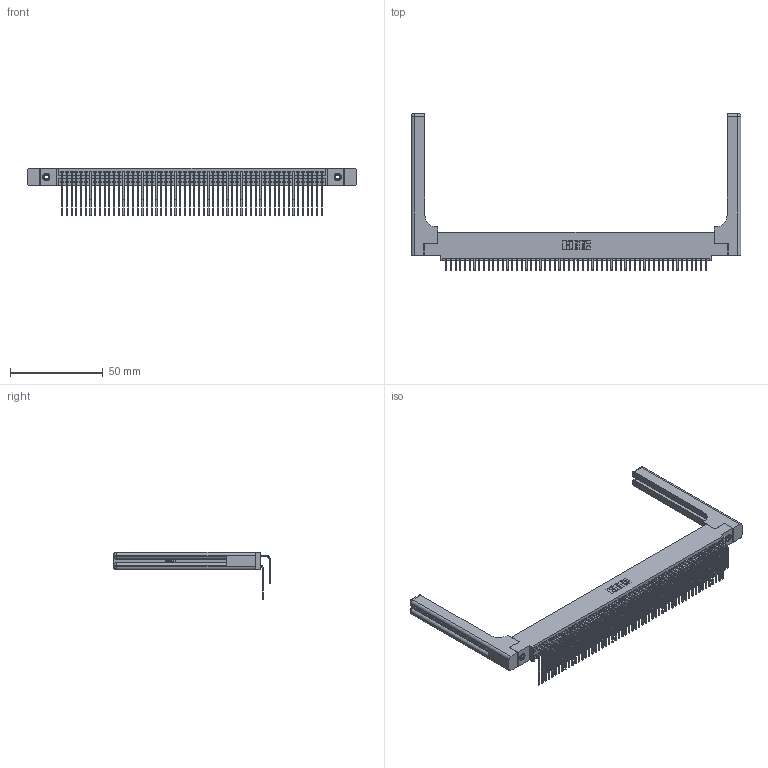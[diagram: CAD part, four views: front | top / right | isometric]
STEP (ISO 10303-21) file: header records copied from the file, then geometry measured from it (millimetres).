
FILE_DESCRIPTION (( 'STEP AP203' ), '1' );
FILE_NAME ('395-112-559-558.STEP', '2019-10-27T16:34:52', ( '' ), ( '' ), 'SwSTEP 2.0', 'SolidWorks 2016', '' );
FILE_SCHEMA (( 'CONFIG_CONTROL_DESIGN' ));
Length unit declared in the file: inch
Products named in the file (6): 345-292-001_558 559 Tail - 1; 345-292-001_559 Tail - 2; 345-250-001_345-250-001-102; 345-220-058_345-220-058; 395-112-559-558; 345 Part_0.110 Offset - 0.156 Dia-TH
Assembly tree (117 placements, depth 2):
  395-112-559-558
    345 Part_0.110 Offset - 0.156 Dia-TH
    345-292-001_558 559 Tail - 1  x56
    345-292-001_559 Tail - 2  x56
    345-250-001_345-250-001-102  x2
    345-220-058_345-220-058  x2
Bounding box: 177.27 x 84.32 x 25.53 mm (x, y, z)
Volume: 26397.7 mm3; surface area: 34953.5 mm2
Topology: 117 solids, 117 shells, 6210 faces, 18379 edges, 12082 vertices
Faces by surface type: plane 4152, cylinder 1998, bspline 36, cone 12, sphere 8, torus 4
Entity records: 49020 total; most frequent: CARTESIAN_POINT 9244, ORIENTED_EDGE 7924, DIRECTION 7038, EDGE_CURVE 3962, VECTOR 3474, LINE 3474, VERTEX_POINT 2630, AXIS2_PLACEMENT_3D 1782
